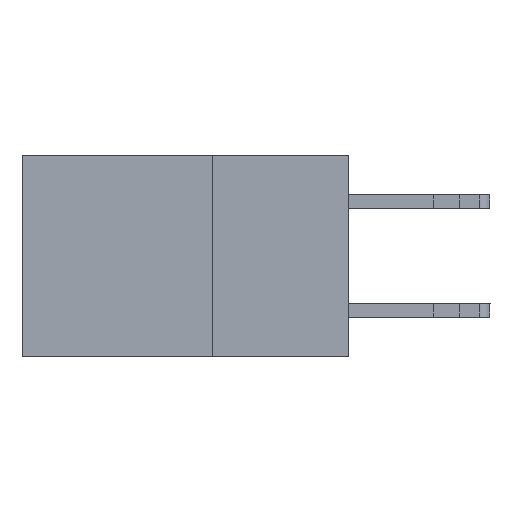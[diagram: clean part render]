
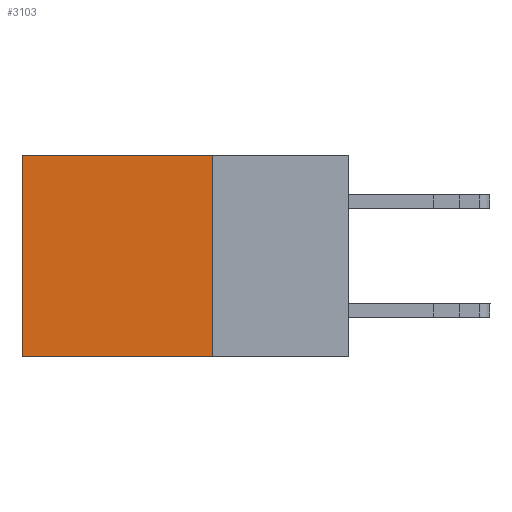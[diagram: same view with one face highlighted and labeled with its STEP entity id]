
A CAD part, left-side view. The second image highlights one B-rep face of the part: STEP entity #3103.
In plain terms, the highlighted planar face has unit normal (-1, 0, 0).
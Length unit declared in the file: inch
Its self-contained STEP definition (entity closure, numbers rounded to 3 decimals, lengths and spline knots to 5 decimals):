
#502 = CARTESIAN_POINT ( 'NONE',  ( 0.2615, 0.6, -0.37 ) ) ;
#717 = DIRECTION ( 'NONE',  ( 0., 0., -1. ) ) ;
#1728 = EDGE_CURVE ( 'NONE', #5499, #4852, #11344, .T. ) ;
#2327 = PLANE ( 'NONE',  #11039 ) ;
#2343 = CARTESIAN_POINT ( 'NONE',  ( 0.2615, 0.25, -0.37 ) ) ;
#2436 = DIRECTION ( 'NONE',  ( 1., 0., 0. ) ) ;
#2545 = ORIENTED_EDGE ( 'NONE', *, *, #10850, .T. ) ;
#2937 = VECTOR ( 'NONE', #9882, 39.37008 ) ;
#3053 = DIRECTION ( 'NONE',  ( 0., 0., -1. ) ) ;
#3103 = ADVANCED_FACE ( 'NONE', ( #6585 ), #2327, .F. ) ;
#3156 = VERTEX_POINT ( 'NONE', #11310 ) ;
#3285 = CARTESIAN_POINT ( 'NONE',  ( 0.2615, 0.25, 0. ) ) ;
#3435 = LINE ( 'NONE', #4405, #6762 ) ;
#4134 = VECTOR ( 'NONE', #8901, 39.37008 ) ;
#4395 = DIRECTION ( 'NONE',  ( 0., 0., -1. ) ) ;
#4405 = CARTESIAN_POINT ( 'NONE',  ( 0.2615, 0.25, -0.37 ) ) ;
#4852 = VERTEX_POINT ( 'NONE', #502 ) ;
#5103 = EDGE_CURVE ( 'NONE', #7673, #5499, #3435, .T. ) ;
#5499 = VERTEX_POINT ( 'NONE', #10798 ) ;
#5541 = EDGE_CURVE ( 'NONE', #7673, #3156, #12662, .T. ) ;
#5956 = ORIENTED_EDGE ( 'NONE', *, *, #1728, .F. ) ;
#6295 = ORIENTED_EDGE ( 'NONE', *, *, #5541, .T. ) ;
#6542 = EDGE_LOOP ( 'NONE', ( #2545, #5956, #11669, #6295 ) ) ;
#6585 = FACE_OUTER_BOUND ( 'NONE', #6542, .T. ) ;
#6762 = VECTOR ( 'NONE', #4395, 39.37008 ) ;
#7673 = VERTEX_POINT ( 'NONE', #3285 ) ;
#8901 = DIRECTION ( 'NONE',  ( 0., 1., 0. ) ) ;
#8953 = CARTESIAN_POINT ( 'NONE',  ( 0.2615, 0.25, 0. ) ) ;
#9676 = CARTESIAN_POINT ( 'NONE',  ( 0.2615, 0.6, -0.37 ) ) ;
#9882 = DIRECTION ( 'NONE',  ( 0., 1., 0. ) ) ;
#10798 = CARTESIAN_POINT ( 'NONE',  ( 0.2615, 0.25, -0.37 ) ) ;
#10850 = EDGE_CURVE ( 'NONE', #3156, #4852, #10983, .T. ) ;
#10983 = LINE ( 'NONE', #9676, #13295 ) ;
#11039 = AXIS2_PLACEMENT_3D ( 'NONE', #2343, #2436, #717 ) ;
#11310 = CARTESIAN_POINT ( 'NONE',  ( 0.2615, 0.6, 0. ) ) ;
#11344 = LINE ( 'NONE', #13544, #2937 ) ;
#11669 = ORIENTED_EDGE ( 'NONE', *, *, #5103, .F. ) ;
#12662 = LINE ( 'NONE', #8953, #4134 ) ;
#13295 = VECTOR ( 'NONE', #3053, 39.37008 ) ;
#13544 = CARTESIAN_POINT ( 'NONE',  ( 0.2615, 0.25, -0.37 ) ) ;
